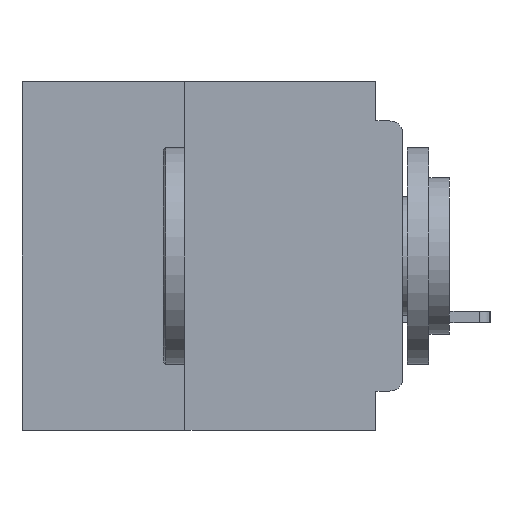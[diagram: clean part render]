
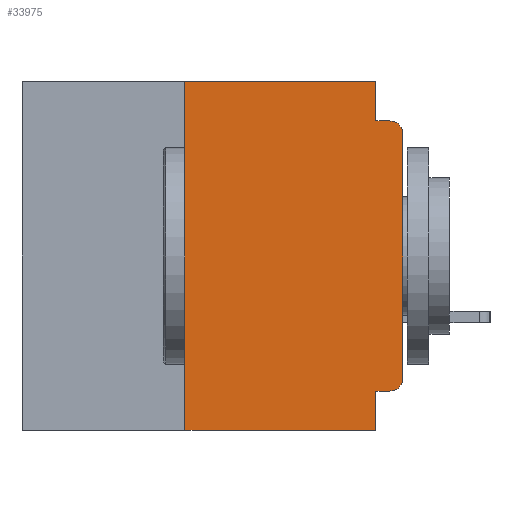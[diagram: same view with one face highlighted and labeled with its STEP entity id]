
A CAD part, left-side view. The second image highlights one B-rep face of the part: STEP entity #33975.
In plain terms, the highlighted planar face has unit normal (-1, 0, 0).
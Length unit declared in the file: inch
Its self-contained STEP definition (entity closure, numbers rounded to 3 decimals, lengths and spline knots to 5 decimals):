
#195 = ORIENTED_EDGE ( 'NONE', *, *, #45330, .F. ) ;
#1063 = CIRCLE ( 'NONE', #4539, 0.015 ) ;
#1374 = EDGE_LOOP ( 'NONE', ( #45616, #16957, #31748, #28008, #27453, #195, #51566, #46713, #34141, #44133 ) ) ;
#1497 = CARTESIAN_POINT ( 'NONE',  ( 0., 0.015, -0.045 ) ) ;
#1715 = EDGE_CURVE ( 'NONE', #41249, #34334, #47774, .T. ) ;
#2861 = EDGE_CURVE ( 'NONE', #17881, #32858, #35620, .T. ) ;
#2923 = CARTESIAN_POINT ( 'NONE',  ( 0., 0., -0.06 ) ) ;
#3452 = CARTESIAN_POINT ( 'NONE',  ( 0., 0., -0.045 ) ) ;
#4539 = AXIS2_PLACEMENT_3D ( 'NONE', #45020, #20701, #49094 ) ;
#5520 = CARTESIAN_POINT ( 'NONE',  ( 0., 0.015, -0.355 ) ) ;
#6197 = VECTOR ( 'NONE', #31338, 39.37008 ) ;
#8495 = EDGE_CURVE ( 'NONE', #21987, #14127, #42662, .T. ) ;
#10521 = VERTEX_POINT ( 'NONE', #2923 ) ;
#10818 = CARTESIAN_POINT ( 'NONE',  ( 0., 0.031, -0.045 ) ) ;
#11940 = CARTESIAN_POINT ( 'NONE',  ( 0., 0.437, 0. ) ) ;
#13742 = CARTESIAN_POINT ( 'NONE',  ( 0., 0.25, -0.4 ) ) ;
#13758 = LINE ( 'NONE', #35208, #46139 ) ;
#14127 = VERTEX_POINT ( 'NONE', #51600 ) ;
#14145 = LINE ( 'NONE', #49601, #31873 ) ;
#14914 = CARTESIAN_POINT ( 'NONE',  ( 0., 0.031, 0. ) ) ;
#15390 = VECTOR ( 'NONE', #16214, 39.37008 ) ;
#15776 = CARTESIAN_POINT ( 'NONE',  ( 0., 0.437, 0. ) ) ;
#15840 = CARTESIAN_POINT ( 'NONE',  ( 0., 0.015, -0.34 ) ) ;
#16004 = DIRECTION ( 'NONE',  ( 0., 0., -1. ) ) ;
#16214 = DIRECTION ( 'NONE',  ( 0., -1., 0. ) ) ;
#16321 = FACE_OUTER_BOUND ( 'NONE', #1374, .T. ) ;
#16486 = CARTESIAN_POINT ( 'NONE',  ( 0., 0.031, -0.355 ) ) ;
#16957 = ORIENTED_EDGE ( 'NONE', *, *, #52098, .T. ) ;
#17881 = VERTEX_POINT ( 'NONE', #10818 ) ;
#19213 = VECTOR ( 'NONE', #32193, 39.37008 ) ;
#19249 = CARTESIAN_POINT ( 'NONE',  ( 0., 0., -0.34 ) ) ;
#19917 = DIRECTION ( 'NONE',  ( 0., 0., -1. ) ) ;
#19971 = CARTESIAN_POINT ( 'NONE',  ( 0., 0.25, -0.4 ) ) ;
#20701 = DIRECTION ( 'NONE',  ( -1., 0., 0. ) ) ;
#21585 = DIRECTION ( 'NONE',  ( 0., 1., 0. ) ) ;
#21987 = VERTEX_POINT ( 'NONE', #16486 ) ;
#23086 = EDGE_CURVE ( 'NONE', #52477, #10521, #38489, .T. ) ;
#25272 = DIRECTION ( 'NONE',  ( 0., -1., 0. ) ) ;
#25672 = DIRECTION ( 'NONE',  ( 0., 0., -1. ) ) ;
#27291 = CARTESIAN_POINT ( 'NONE',  ( 0., 0., 0. ) ) ;
#27453 = ORIENTED_EDGE ( 'NONE', *, *, #1715, .F. ) ;
#28008 = ORIENTED_EDGE ( 'NONE', *, *, #44463, .F. ) ;
#28703 = LINE ( 'NONE', #19971, #19213 ) ;
#31338 = DIRECTION ( 'NONE',  ( 0., 0., 1. ) ) ;
#31748 = ORIENTED_EDGE ( 'NONE', *, *, #2861, .F. ) ;
#31795 = CARTESIAN_POINT ( 'NONE',  ( 0., 0.25, 0. ) ) ;
#31873 = VECTOR ( 'NONE', #25272, 39.37008 ) ;
#32193 = DIRECTION ( 'NONE',  ( 0., 0., 1. ) ) ;
#32858 = VERTEX_POINT ( 'NONE', #1497 ) ;
#33975 = ADVANCED_FACE ( 'NONE', ( #16321 ), #36186, .F. ) ;
#34141 = ORIENTED_EDGE ( 'NONE', *, *, #46823, .F. ) ;
#34334 = VERTEX_POINT ( 'NONE', #14914 ) ;
#35208 = CARTESIAN_POINT ( 'NONE',  ( 0., 0.031, 0. ) ) ;
#35620 = LINE ( 'NONE', #3452, #45188 ) ;
#35725 = EDGE_CURVE ( 'NONE', #43586, #52477, #44682, .T. ) ;
#36127 = VECTOR ( 'NONE', #21585, 39.37008 ) ;
#36186 = PLANE ( 'NONE',  #47126 ) ;
#38489 = LINE ( 'NONE', #27291, #6197 ) ;
#39281 = DIRECTION ( 'NONE',  ( 0., 0., -1. ) ) ;
#39983 = DIRECTION ( 'NONE',  ( 0., -1., 0. ) ) ;
#40273 = DIRECTION ( 'NONE',  ( 1., 0., 0. ) ) ;
#41249 = VERTEX_POINT ( 'NONE', #31795 ) ;
#41370 = VECTOR ( 'NONE', #25672, 39.37008 ) ;
#42662 = LINE ( 'NONE', #45917, #41370 ) ;
#43022 = VERTEX_POINT ( 'NONE', #13742 ) ;
#43586 = VERTEX_POINT ( 'NONE', #5520 ) ;
#43779 = AXIS2_PLACEMENT_3D ( 'NONE', #15840, #44225, #19917 ) ;
#44133 = ORIENTED_EDGE ( 'NONE', *, *, #35725, .T. ) ;
#44225 = DIRECTION ( 'NONE',  ( -1., 0., 0. ) ) ;
#44463 = EDGE_CURVE ( 'NONE', #34334, #17881, #13758, .T. ) ;
#44682 = CIRCLE ( 'NONE', #43779, 0.015 ) ;
#45020 = CARTESIAN_POINT ( 'NONE',  ( 0., 0.015, -0.06 ) ) ;
#45188 = VECTOR ( 'NONE', #39983, 39.37008 ) ;
#45330 = EDGE_CURVE ( 'NONE', #43022, #41249, #28703, .T. ) ;
#45478 = EDGE_CURVE ( 'NONE', #43022, #14127, #14145, .T. ) ;
#45616 = ORIENTED_EDGE ( 'NONE', *, *, #23086, .T. ) ;
#45913 = CARTESIAN_POINT ( 'NONE',  ( 0., 0., -0.355 ) ) ;
#45917 = CARTESIAN_POINT ( 'NONE',  ( 0., 0.031, -0.4 ) ) ;
#46139 = VECTOR ( 'NONE', #39281, 39.37008 ) ;
#46713 = ORIENTED_EDGE ( 'NONE', *, *, #8495, .F. ) ;
#46823 = EDGE_CURVE ( 'NONE', #43586, #21987, #46972, .T. ) ;
#46972 = LINE ( 'NONE', #45913, #36127 ) ;
#47126 = AXIS2_PLACEMENT_3D ( 'NONE', #11940, #40273, #16004 ) ;
#47774 = LINE ( 'NONE', #15776, #15390 ) ;
#49094 = DIRECTION ( 'NONE',  ( 0., 0., -1. ) ) ;
#49601 = CARTESIAN_POINT ( 'NONE',  ( 0., 0.437, -0.4 ) ) ;
#51566 = ORIENTED_EDGE ( 'NONE', *, *, #45478, .T. ) ;
#51600 = CARTESIAN_POINT ( 'NONE',  ( 0., 0.031, -0.4 ) ) ;
#52098 = EDGE_CURVE ( 'NONE', #10521, #32858, #1063, .T. ) ;
#52477 = VERTEX_POINT ( 'NONE', #19249 ) ;
